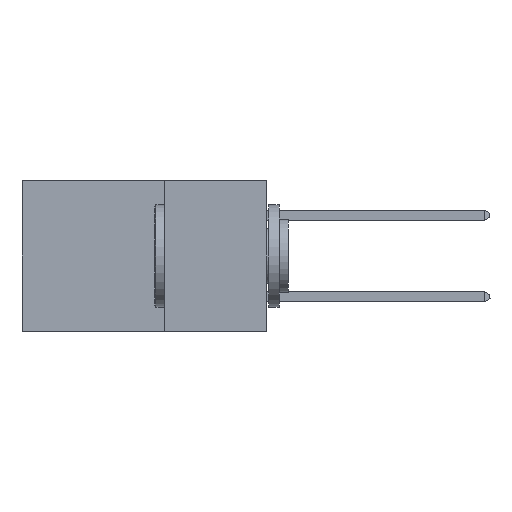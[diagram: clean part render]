
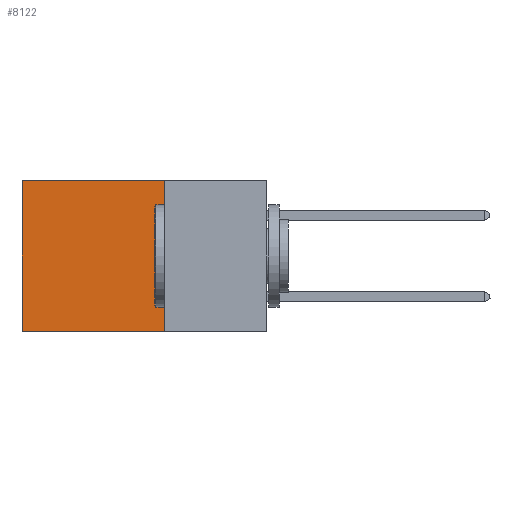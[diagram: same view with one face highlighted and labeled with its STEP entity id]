
A CAD part, left-side view. The second image highlights one B-rep face of the part: STEP entity #8122.
In plain terms, the highlighted planar face has unit normal (-1, 0, 0).
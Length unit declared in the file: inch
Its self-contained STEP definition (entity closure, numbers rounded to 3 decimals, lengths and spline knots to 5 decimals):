
#1563 = CARTESIAN_POINT ( 'NONE',  ( 0.2875, 0.6, 0. ) ) ;
#3193 = CARTESIAN_POINT ( 'NONE',  ( 0.2875, 0.6, 0. ) ) ;
#4513 = VERTEX_POINT ( 'NONE', #18787 ) ;
#5021 = CARTESIAN_POINT ( 'NONE',  ( 0.2875, 0.25, 0. ) ) ;
#5379 = PLANE ( 'NONE',  #10873 ) ;
#5872 = VECTOR ( 'NONE', #14080, 39.37008 ) ;
#6318 = VECTOR ( 'NONE', #15148, 39.37008 ) ;
#6336 = EDGE_CURVE ( 'NONE', #20041, #4513, #21067, .T. ) ;
#6714 = ORIENTED_EDGE ( 'NONE', *, *, #26510, .T. ) ;
#7447 = LINE ( 'NONE', #10278, #14334 ) ;
#7894 = CARTESIAN_POINT ( 'NONE',  ( 0.2875, 0.25, 0. ) ) ;
#8122 = ADVANCED_FACE ( 'NONE', ( #22253 ), #5379, .F. ) ;
#9891 = CARTESIAN_POINT ( 'NONE',  ( 0.2875, 0.6, -0.37 ) ) ;
#10278 = CARTESIAN_POINT ( 'NONE',  ( 0.2875, 0.25, -0.37 ) ) ;
#10858 = VERTEX_POINT ( 'NONE', #9891 ) ;
#10873 = AXIS2_PLACEMENT_3D ( 'NONE', #7894, #16209, #11807 ) ;
#11807 = DIRECTION ( 'NONE',  ( 0., 0., -1. ) ) ;
#13631 = ORIENTED_EDGE ( 'NONE', *, *, #6336, .F. ) ;
#14080 = DIRECTION ( 'NONE',  ( 0., 0., -1. ) ) ;
#14334 = VECTOR ( 'NONE', #17258, 39.37008 ) ;
#15148 = DIRECTION ( 'NONE',  ( 0., 1., 0. ) ) ;
#15497 = LINE ( 'NONE', #25535, #6318 ) ;
#15779 = ORIENTED_EDGE ( 'NONE', *, *, #21480, .T. ) ;
#16209 = DIRECTION ( 'NONE',  ( 1., 0., 0. ) ) ;
#16820 = EDGE_CURVE ( 'NONE', #4513, #10858, #7447, .T. ) ;
#17160 = VECTOR ( 'NONE', #25886, 39.37008 ) ;
#17258 = DIRECTION ( 'NONE',  ( 0., 1., 0. ) ) ;
#18787 = CARTESIAN_POINT ( 'NONE',  ( 0.2875, 0.25, -0.37 ) ) ;
#20041 = VERTEX_POINT ( 'NONE', #23780 ) ;
#20847 = EDGE_LOOP ( 'NONE', ( #15779, #21666, #13631, #6714 ) ) ;
#21067 = LINE ( 'NONE', #5021, #17160 ) ;
#21270 = LINE ( 'NONE', #1563, #5872 ) ;
#21480 = EDGE_CURVE ( 'NONE', #26803, #10858, #21270, .T. ) ;
#21666 = ORIENTED_EDGE ( 'NONE', *, *, #16820, .F. ) ;
#22253 = FACE_OUTER_BOUND ( 'NONE', #20847, .T. ) ;
#23780 = CARTESIAN_POINT ( 'NONE',  ( 0.2875, 0.25, 0. ) ) ;
#25535 = CARTESIAN_POINT ( 'NONE',  ( 0.2875, 0.25, 0. ) ) ;
#25886 = DIRECTION ( 'NONE',  ( 0., 0., -1. ) ) ;
#26510 = EDGE_CURVE ( 'NONE', #20041, #26803, #15497, .T. ) ;
#26803 = VERTEX_POINT ( 'NONE', #3193 ) ;
